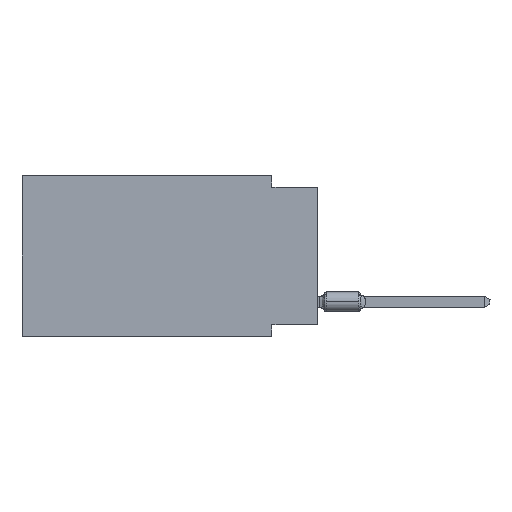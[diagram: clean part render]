
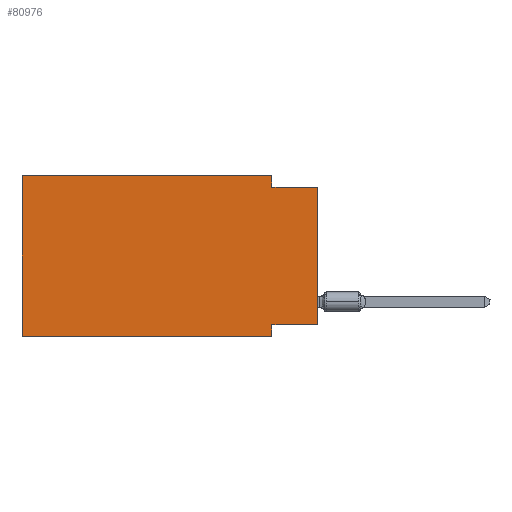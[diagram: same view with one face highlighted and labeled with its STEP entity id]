
A CAD part, left-side view. The second image highlights one B-rep face of the part: STEP entity #80976.
In plain terms, the highlighted planar face has unit normal (-1, 0, 0).
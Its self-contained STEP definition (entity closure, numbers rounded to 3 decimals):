
#461 = EDGE_CURVE ( 'NONE', #80840, #91994, #59689, .T. ) ;
#1789 = DIRECTION ( 'NONE',  ( 0., 0., -1. ) ) ;
#2571 = LINE ( 'NONE', #55834, #107119 ) ;
#3787 = EDGE_CURVE ( 'NONE', #29578, #91994, #70299, .T. ) ;
#4427 = DIRECTION ( 'NONE',  ( 0., 0., -1. ) ) ;
#6798 = ORIENTED_EDGE ( 'NONE', *, *, #103943, .T. ) ;
#7023 = ORIENTED_EDGE ( 'NONE', *, *, #3787, .T. ) ;
#7084 = CARTESIAN_POINT ( 'NONE',  ( 0., 2.54, -0.635 ) ) ;
#10771 = VECTOR ( 'NONE', #17939, 1000. ) ;
#15897 = EDGE_CURVE ( 'NONE', #63323, #18765, #79507, .T. ) ;
#16019 = CARTESIAN_POINT ( 'NONE',  ( 0., 16.383, 0. ) ) ;
#17939 = DIRECTION ( 'NONE',  ( 0., 0., 1. ) ) ;
#18424 = LINE ( 'NONE', #53359, #20202 ) ;
#18555 = ORIENTED_EDGE ( 'NONE', *, *, #15897, .F. ) ;
#18765 = VERTEX_POINT ( 'NONE', #19576 ) ;
#19576 = CARTESIAN_POINT ( 'NONE',  ( 0., 2.54, 0. ) ) ;
#20202 = VECTOR ( 'NONE', #1789, 1000. ) ;
#20304 = ORIENTED_EDGE ( 'NONE', *, *, #59723, .F. ) ;
#21621 = CARTESIAN_POINT ( 'NONE',  ( 0., 16.383, 0. ) ) ;
#26797 = DIRECTION ( 'NONE',  ( 0., -1., 0. ) ) ;
#26802 = VECTOR ( 'NONE', #56413, 1000. ) ;
#29211 = CARTESIAN_POINT ( 'NONE',  ( 0., 0., -0.635 ) ) ;
#29578 = VERTEX_POINT ( 'NONE', #99260 ) ;
#30086 = LINE ( 'NONE', #65002, #26802 ) ;
#32409 = VECTOR ( 'NONE', #94627, 1000. ) ;
#33788 = VERTEX_POINT ( 'NONE', #7084 ) ;
#37072 = EDGE_CURVE ( 'NONE', #18765, #33788, #18424, .T. ) ;
#37532 = DIRECTION ( 'NONE',  ( 0., 0., 1. ) ) ;
#37780 = CARTESIAN_POINT ( 'NONE',  ( 0., 2.54, -8.89 ) ) ;
#38212 = VECTOR ( 'NONE', #85869, 1000. ) ;
#38394 = CARTESIAN_POINT ( 'NONE',  ( 0., 0., -0.635 ) ) ;
#41442 = VECTOR ( 'NONE', #109365, 1000. ) ;
#41737 = VECTOR ( 'NONE', #26797, 1000. ) ;
#43331 = CARTESIAN_POINT ( 'NONE',  ( 0., 0., -8.255 ) ) ;
#43360 = EDGE_CURVE ( 'NONE', #29578, #63323, #52878, .T. ) ;
#46268 = DIRECTION ( 'NONE',  ( 1., 0., 0. ) ) ;
#48182 = ORIENTED_EDGE ( 'NONE', *, *, #37072, .F. ) ;
#50708 = ORIENTED_EDGE ( 'NONE', *, *, #461, .F. ) ;
#52878 = LINE ( 'NONE', #78641, #10771 ) ;
#53359 = CARTESIAN_POINT ( 'NONE',  ( 0., 2.54, 0. ) ) ;
#55834 = CARTESIAN_POINT ( 'NONE',  ( 0., 0., 0. ) ) ;
#56413 = DIRECTION ( 'NONE',  ( 0., 1., 0. ) ) ;
#56685 = LINE ( 'NONE', #29211, #41442 ) ;
#59689 = LINE ( 'NONE', #104339, #32409 ) ;
#59723 = EDGE_CURVE ( 'NONE', #82970, #80840, #30086, .T. ) ;
#63323 = VERTEX_POINT ( 'NONE', #104672 ) ;
#65002 = CARTESIAN_POINT ( 'NONE',  ( 0., 0., -8.255 ) ) ;
#65493 = EDGE_LOOP ( 'NONE', ( #6798, #68821, #48182, #18555, #103934, #7023, #50708, #20304 ) ) ;
#68821 = ORIENTED_EDGE ( 'NONE', *, *, #103039, .F. ) ;
#70299 = LINE ( 'NONE', #105237, #41737 ) ;
#72944 = VERTEX_POINT ( 'NONE', #38394 ) ;
#73730 = FACE_OUTER_BOUND ( 'NONE', #65493, .T. ) ;
#78641 = CARTESIAN_POINT ( 'NONE',  ( 0., 16.383, 0. ) ) ;
#79507 = LINE ( 'NONE', #16019, #38212 ) ;
#80840 = VERTEX_POINT ( 'NONE', #84146 ) ;
#80976 = ADVANCED_FACE ( 'NONE', ( #73730 ), #91468, .F. ) ;
#82970 = VERTEX_POINT ( 'NONE', #43331 ) ;
#84146 = CARTESIAN_POINT ( 'NONE',  ( 0., 2.54, -8.255 ) ) ;
#84753 = AXIS2_PLACEMENT_3D ( 'NONE', #21621, #46268, #4427 ) ;
#85869 = DIRECTION ( 'NONE',  ( 0., -1., 0. ) ) ;
#91468 = PLANE ( 'NONE',  #84753 ) ;
#91994 = VERTEX_POINT ( 'NONE', #37780 ) ;
#94627 = DIRECTION ( 'NONE',  ( 0., 0., -1. ) ) ;
#99260 = CARTESIAN_POINT ( 'NONE',  ( 0., 16.383, -8.89 ) ) ;
#103039 = EDGE_CURVE ( 'NONE', #33788, #72944, #56685, .T. ) ;
#103934 = ORIENTED_EDGE ( 'NONE', *, *, #43360, .F. ) ;
#103943 = EDGE_CURVE ( 'NONE', #82970, #72944, #2571, .T. ) ;
#104339 = CARTESIAN_POINT ( 'NONE',  ( 0., 2.54, -8.89 ) ) ;
#104672 = CARTESIAN_POINT ( 'NONE',  ( 0., 16.383, 0. ) ) ;
#105237 = CARTESIAN_POINT ( 'NONE',  ( 0., 16.383, -8.89 ) ) ;
#107119 = VECTOR ( 'NONE', #37532, 1000. ) ;
#109365 = DIRECTION ( 'NONE',  ( 0., -1., 0. ) ) ;
